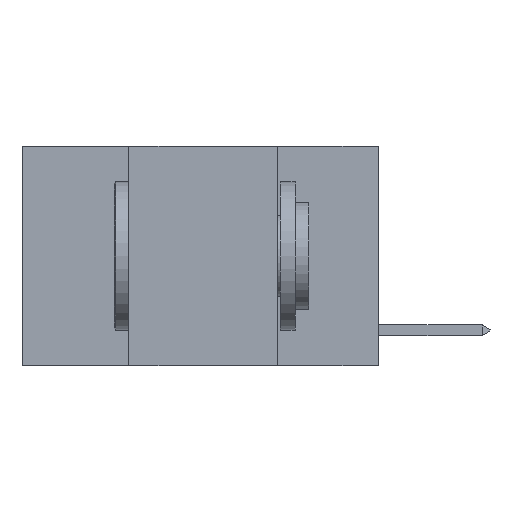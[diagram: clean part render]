
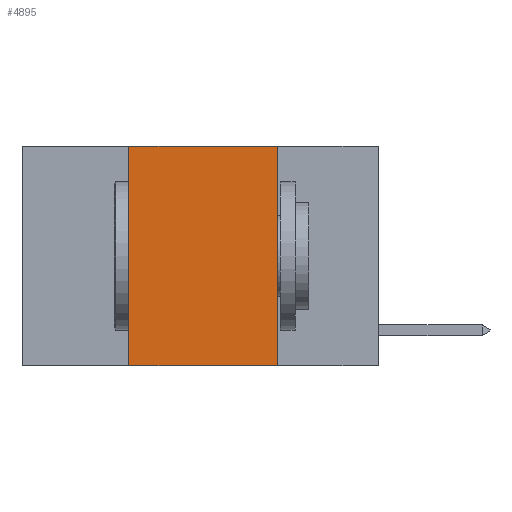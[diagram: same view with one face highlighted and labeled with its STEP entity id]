
A CAD part, left-side view. The second image highlights one B-rep face of the part: STEP entity #4895.
In plain terms, the highlighted planar face has unit normal (-1, 0, 0).
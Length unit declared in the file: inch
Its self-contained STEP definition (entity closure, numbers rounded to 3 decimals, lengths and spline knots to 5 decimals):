
#280 = DIRECTION ( 'NONE',  ( 0., 0., -1. ) ) ;
#316 = DIRECTION ( 'NONE',  ( 1., 0., 0. ) ) ;
#351 = PLANE ( 'NONE',  #911 ) ;
#492 = CARTESIAN_POINT ( 'NONE',  ( 0., 0.6, 0. ) ) ;
#577 = EDGE_LOOP ( 'NONE', ( #5274, #5762, #5909, #5949 ) ) ;
#911 = AXIS2_PLACEMENT_3D ( 'NONE', #492, #316, #280 ) ;
#1032 = VERTEX_POINT ( 'NONE', #7495 ) ;
#1331 = CARTESIAN_POINT ( 'NONE',  ( 0., 0.17, 0. ) ) ;
#1539 = VERTEX_POINT ( 'NONE', #5983 ) ;
#1911 = DIRECTION ( 'NONE',  ( 0., -1., 0. ) ) ;
#1927 = CARTESIAN_POINT ( 'NONE',  ( 0., 0.6, 0. ) ) ;
#2183 = CARTESIAN_POINT ( 'NONE',  ( 0., 0.17, -0.37 ) ) ;
#3371 = CARTESIAN_POINT ( 'NONE',  ( 0., 0.42, -0.37 ) ) ;
#3423 = FACE_OUTER_BOUND ( 'NONE', #577, .T. ) ;
#3868 = VERTEX_POINT ( 'NONE', #3371 ) ;
#3884 = VECTOR ( 'NONE', #1911, 39.37008 ) ;
#4895 = ADVANCED_FACE ( 'NONE', ( #3423 ), #351, .F. ) ;
#5274 = ORIENTED_EDGE ( 'NONE', *, *, #6687, .F. ) ;
#5338 = VECTOR ( 'NONE', #8681, 39.37008 ) ;
#5745 = LINE ( 'NONE', #8716, #5338 ) ;
#5762 = ORIENTED_EDGE ( 'NONE', *, *, #6387, .F. ) ;
#5795 = VECTOR ( 'NONE', #8790, 39.37008 ) ;
#5909 = ORIENTED_EDGE ( 'NONE', *, *, #6688, .F. ) ;
#5949 = ORIENTED_EDGE ( 'NONE', *, *, #6696, .T. ) ;
#5983 = CARTESIAN_POINT ( 'NONE',  ( 0., 0.17, 0. ) ) ;
#6018 = LINE ( 'NONE', #1331, #5795 ) ;
#6240 = VECTOR ( 'NONE', #8724, 39.37008 ) ;
#6387 = EDGE_CURVE ( 'NONE', #1032, #1539, #6953, .T. ) ;
#6589 = LINE ( 'NONE', #8886, #6240 ) ;
#6687 = EDGE_CURVE ( 'NONE', #1539, #7183, #6018, .T. ) ;
#6688 = EDGE_CURVE ( 'NONE', #3868, #1032, #6589, .T. ) ;
#6696 = EDGE_CURVE ( 'NONE', #3868, #7183, #5745, .T. ) ;
#6953 = LINE ( 'NONE', #1927, #3884 ) ;
#7183 = VERTEX_POINT ( 'NONE', #2183 ) ;
#7495 = CARTESIAN_POINT ( 'NONE',  ( 0., 0.42, 0. ) ) ;
#8681 = DIRECTION ( 'NONE',  ( 0., -1., 0. ) ) ;
#8716 = CARTESIAN_POINT ( 'NONE',  ( 0., 0.6, -0.37 ) ) ;
#8724 = DIRECTION ( 'NONE',  ( 0., 0., 1. ) ) ;
#8790 = DIRECTION ( 'NONE',  ( 0., 0., -1. ) ) ;
#8886 = CARTESIAN_POINT ( 'NONE',  ( 0., 0.42, 0. ) ) ;
